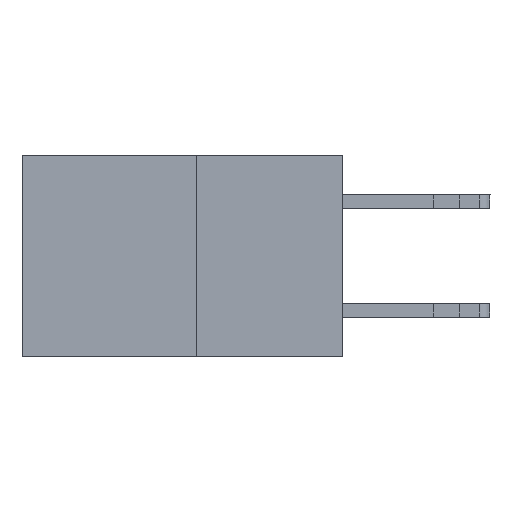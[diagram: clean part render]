
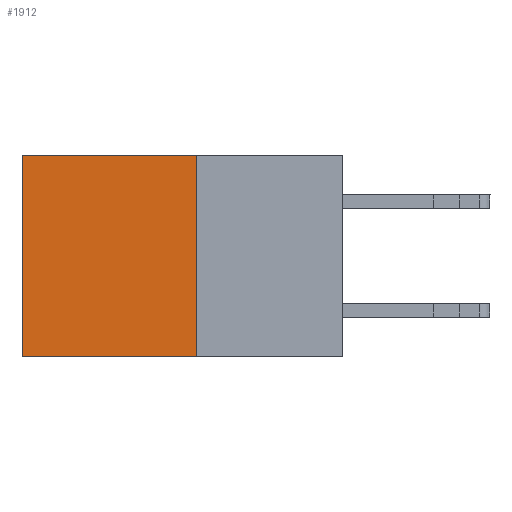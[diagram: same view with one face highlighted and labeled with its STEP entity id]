
A CAD part, left-side view. The second image highlights one B-rep face of the part: STEP entity #1912.
In plain terms, the highlighted planar face has unit normal (-1, 0, 0).
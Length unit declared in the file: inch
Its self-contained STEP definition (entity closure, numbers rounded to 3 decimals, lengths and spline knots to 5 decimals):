
#273 = EDGE_CURVE ( 'NONE', #4281, #5460, #13458, .T. ) ;
#1912 = ADVANCED_FACE ( 'NONE', ( #2840 ), #14594, .F. ) ;
#2211 = DIRECTION ( 'NONE',  ( 0., 1., 0. ) ) ;
#2702 = EDGE_CURVE ( 'NONE', #5460, #9051, #3746, .T. ) ;
#2790 = VECTOR ( 'NONE', #2211, 39.37008 ) ;
#2840 = FACE_OUTER_BOUND ( 'NONE', #11656, .T. ) ;
#2947 = DIRECTION ( 'NONE',  ( 0., 0., -1. ) ) ;
#3746 = LINE ( 'NONE', #15296, #19989 ) ;
#4095 = CARTESIAN_POINT ( 'NONE',  ( 0.277, 0.59, -0.37 ) ) ;
#4141 = ORIENTED_EDGE ( 'NONE', *, *, #14505, .T. ) ;
#4281 = VERTEX_POINT ( 'NONE', #16201 ) ;
#4301 = ORIENTED_EDGE ( 'NONE', *, *, #273, .F. ) ;
#4400 = EDGE_CURVE ( 'NONE', #4281, #16217, #5500, .T. ) ;
#5110 = DIRECTION ( 'NONE',  ( 0., 0., -1. ) ) ;
#5337 = CARTESIAN_POINT ( 'NONE',  ( 0.277, 0.27, -0.37 ) ) ;
#5339 = CARTESIAN_POINT ( 'NONE',  ( 0.277, 0.59, 0. ) ) ;
#5460 = VERTEX_POINT ( 'NONE', #5666 ) ;
#5500 = LINE ( 'NONE', #15410, #2790 ) ;
#5666 = CARTESIAN_POINT ( 'NONE',  ( 0.277, 0.27, -0.37 ) ) ;
#5683 = LINE ( 'NONE', #10419, #17070 ) ;
#6250 = CARTESIAN_POINT ( 'NONE',  ( 0.277, 0.27, -0.37 ) ) ;
#7221 = DIRECTION ( 'NONE',  ( 0., 0., -1. ) ) ;
#9051 = VERTEX_POINT ( 'NONE', #4095 ) ;
#10419 = CARTESIAN_POINT ( 'NONE',  ( 0.277, 0.59, -0.37 ) ) ;
#11656 = EDGE_LOOP ( 'NONE', ( #4141, #15167, #4301, #15602 ) ) ;
#13458 = LINE ( 'NONE', #5337, #19385 ) ;
#14505 = EDGE_CURVE ( 'NONE', #16217, #9051, #5683, .T. ) ;
#14594 = PLANE ( 'NONE',  #15164 ) ;
#15164 = AXIS2_PLACEMENT_3D ( 'NONE', #6250, #19677, #2947 ) ;
#15167 = ORIENTED_EDGE ( 'NONE', *, *, #2702, .F. ) ;
#15296 = CARTESIAN_POINT ( 'NONE',  ( 0.277, 0.27, -0.37 ) ) ;
#15410 = CARTESIAN_POINT ( 'NONE',  ( 0.277, 0.27, 0. ) ) ;
#15602 = ORIENTED_EDGE ( 'NONE', *, *, #4400, .T. ) ;
#16201 = CARTESIAN_POINT ( 'NONE',  ( 0.277, 0.27, 0. ) ) ;
#16217 = VERTEX_POINT ( 'NONE', #5339 ) ;
#17070 = VECTOR ( 'NONE', #7221, 39.37008 ) ;
#18936 = DIRECTION ( 'NONE',  ( 0., 1., 0. ) ) ;
#19385 = VECTOR ( 'NONE', #5110, 39.37008 ) ;
#19677 = DIRECTION ( 'NONE',  ( 1., 0., 0. ) ) ;
#19989 = VECTOR ( 'NONE', #18936, 39.37008 ) ;
